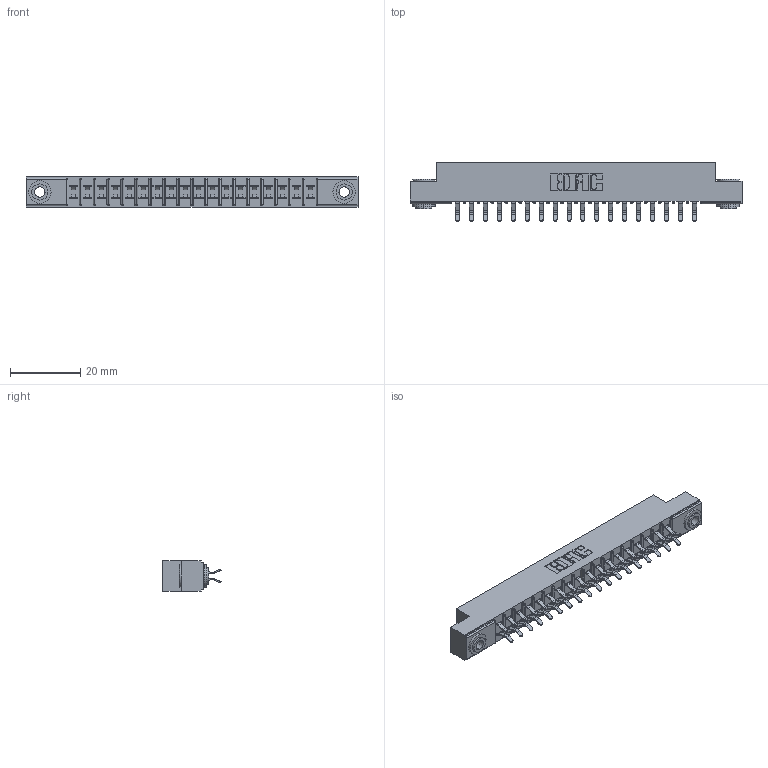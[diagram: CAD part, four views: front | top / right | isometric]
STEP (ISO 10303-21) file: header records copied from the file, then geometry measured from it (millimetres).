
FILE_DESCRIPTION (( 'STEP AP203' ), '1' );
FILE_NAME ('315-036-556-203.STEP', '2019-09-10T16:17:31', ( '' ), ( '' ), 'SwSTEP 2.0', 'SolidWorks 2016', '' );
FILE_SCHEMA (( 'CONFIG_CONTROL_DESIGN' ));
Length unit declared in the file: inch
Products named in the file (4): 305-290-001_556; 305 Part_.156 Dia; 345-250-002_345-250-002-102; 315-036-556-203
Assembly tree (39 placements, depth 2):
  315-036-556-203
    305 Part_.156 Dia
    305-290-001_556  x36
    345-250-002_345-250-002-102  x2
Bounding box: 94.34 x 16.64 x 8.71 mm (x, y, z)
Volume: 5922.4 mm3; surface area: 11197.9 mm2
Topology: 39 solids, 39 shells, 2184 faces, 6242 edges, 4060 vertices
Faces by surface type: plane 1208, cylinder 896, sphere 72, cone 8
Entity records: 23698 total; most frequent: CARTESIAN_POINT 3905, ORIENTED_EDGE 3864, DIRECTION 3816, EDGE_CURVE 1932, VECTOR 1522, LINE 1522, VERTEX_POINT 1236, AXIS2_PLACEMENT_3D 1147
